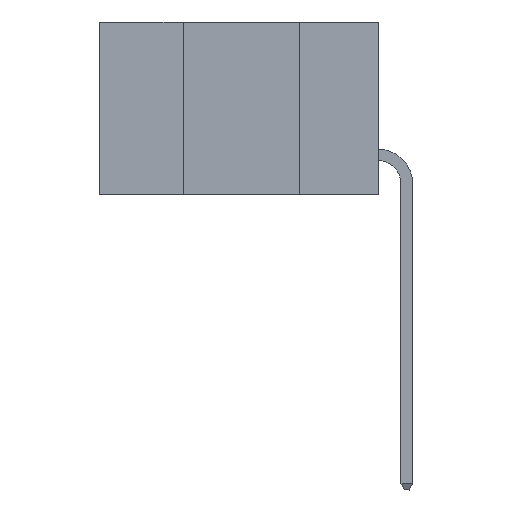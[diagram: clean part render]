
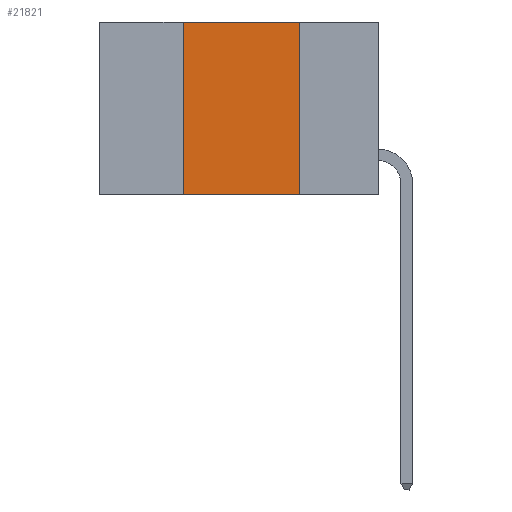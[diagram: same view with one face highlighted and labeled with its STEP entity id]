
A CAD part, left-side view. The second image highlights one B-rep face of the part: STEP entity #21821.
In plain terms, the highlighted planar face has unit normal (-1, 0, 0).
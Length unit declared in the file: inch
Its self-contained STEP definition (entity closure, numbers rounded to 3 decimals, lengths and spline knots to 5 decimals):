
#395 = DIRECTION ( 'NONE',  ( 0., -1., 0. ) ) ;
#2378 = VECTOR ( 'NONE', #14645, 39.37008 ) ;
#2422 = DIRECTION ( 'NONE',  ( 0., 0., -1. ) ) ;
#2805 = LINE ( 'NONE', #16688, #4694 ) ;
#3308 = CARTESIAN_POINT ( 'NONE',  ( 0., 0.42, -0.37 ) ) ;
#3356 = CARTESIAN_POINT ( 'NONE',  ( 0., 0.6, 0. ) ) ;
#3579 = VECTOR ( 'NONE', #395, 39.37008 ) ;
#3610 = VERTEX_POINT ( 'NONE', #22507 ) ;
#4229 = PLANE ( 'NONE',  #21662 ) ;
#4417 = ORIENTED_EDGE ( 'NONE', *, *, #11231, .F. ) ;
#4694 = VECTOR ( 'NONE', #12696, 39.37008 ) ;
#7677 = ORIENTED_EDGE ( 'NONE', *, *, #7996, .F. ) ;
#7968 = FACE_OUTER_BOUND ( 'NONE', #13130, .T. ) ;
#7996 = EDGE_CURVE ( 'NONE', #20046, #3610, #12601, .T. ) ;
#8210 = CARTESIAN_POINT ( 'NONE',  ( 0., 0.6, 0. ) ) ;
#10739 = VECTOR ( 'NONE', #24572, 39.37008 ) ;
#11231 = EDGE_CURVE ( 'NONE', #3610, #21184, #2805, .T. ) ;
#11824 = DIRECTION ( 'NONE',  ( 1., 0., 0. ) ) ;
#12090 = ORIENTED_EDGE ( 'NONE', *, *, #17127, .F. ) ;
#12601 = LINE ( 'NONE', #3356, #10739 ) ;
#12696 = DIRECTION ( 'NONE',  ( 0., 0., -1. ) ) ;
#13130 = EDGE_LOOP ( 'NONE', ( #4417, #7677, #12090, #21281 ) ) ;
#14495 = CARTESIAN_POINT ( 'NONE',  ( 0., 0.42, 0. ) ) ;
#14520 = LINE ( 'NONE', #16574, #2378 ) ;
#14645 = DIRECTION ( 'NONE',  ( 0., 0., 1. ) ) ;
#15322 = CARTESIAN_POINT ( 'NONE',  ( 0., 0.17, -0.37 ) ) ;
#16200 = CARTESIAN_POINT ( 'NONE',  ( 0., 0.6, -0.37 ) ) ;
#16574 = CARTESIAN_POINT ( 'NONE',  ( 0., 0.42, -0.37 ) ) ;
#16688 = CARTESIAN_POINT ( 'NONE',  ( 0., 0.17, -0.37 ) ) ;
#17127 = EDGE_CURVE ( 'NONE', #20233, #20046, #14520, .T. ) ;
#18033 = LINE ( 'NONE', #16200, #3579 ) ;
#20046 = VERTEX_POINT ( 'NONE', #14495 ) ;
#20233 = VERTEX_POINT ( 'NONE', #3308 ) ;
#21184 = VERTEX_POINT ( 'NONE', #15322 ) ;
#21281 = ORIENTED_EDGE ( 'NONE', *, *, #22617, .T. ) ;
#21662 = AXIS2_PLACEMENT_3D ( 'NONE', #8210, #11824, #2422 ) ;
#21821 = ADVANCED_FACE ( 'NONE', ( #7968 ), #4229, .F. ) ;
#22507 = CARTESIAN_POINT ( 'NONE',  ( 0., 0.17, 0. ) ) ;
#22617 = EDGE_CURVE ( 'NONE', #20233, #21184, #18033, .T. ) ;
#24572 = DIRECTION ( 'NONE',  ( 0., -1., 0. ) ) ;
